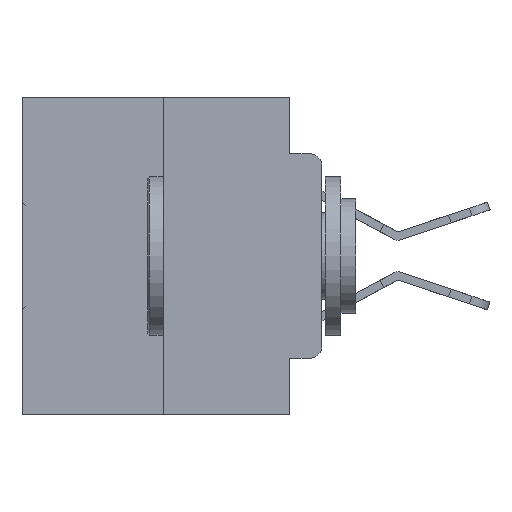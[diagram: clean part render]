
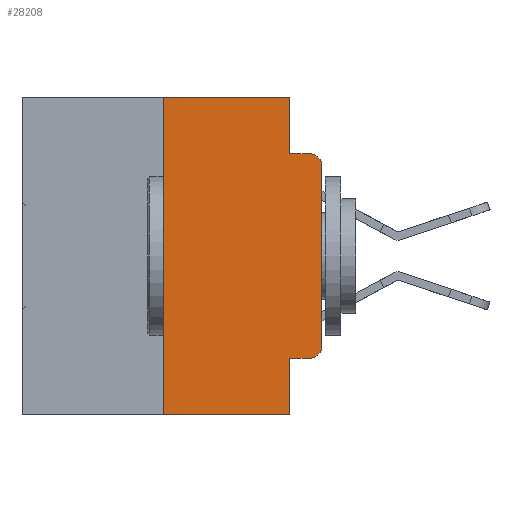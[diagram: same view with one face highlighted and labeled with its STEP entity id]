
A CAD part, left-side view. The second image highlights one B-rep face of the part: STEP entity #28208.
In plain terms, the highlighted planar face has unit normal (-1, 0, 0).
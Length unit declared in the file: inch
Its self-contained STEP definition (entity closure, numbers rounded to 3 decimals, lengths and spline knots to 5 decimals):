
#114 = DIRECTION ( 'NONE',  ( 0., 0., -1. ) ) ;
#362 = EDGE_CURVE ( 'NONE', #10582, #13697, #19929, .T. ) ;
#830 = VERTEX_POINT ( 'NONE', #8700 ) ;
#1329 = LINE ( 'NONE', #29968, #14332 ) ;
#1713 = VERTEX_POINT ( 'NONE', #24439 ) ;
#2024 = CARTESIAN_POINT ( 'NONE',  ( 0., 0., -0.3915 ) ) ;
#2115 = DIRECTION ( 'NONE',  ( 0., 0., -1. ) ) ;
#2784 = EDGE_CURVE ( 'NONE', #21373, #20872, #1329, .T. ) ;
#3033 = DIRECTION ( 'NONE',  ( 1., 0., 0. ) ) ;
#3530 = CARTESIAN_POINT ( 'NONE',  ( 0., 0.051, 0. ) ) ;
#3586 = CARTESIAN_POINT ( 'NONE',  ( 0., 0.051, -0.0885 ) ) ;
#3989 = LINE ( 'NONE', #27292, #23705 ) ;
#3999 = CARTESIAN_POINT ( 'NONE',  ( 0., 0.051, -0.4115 ) ) ;
#5716 = VECTOR ( 'NONE', #10971, 39.37008 ) ;
#5851 = CIRCLE ( 'NONE', #15450, 0.02 ) ;
#6141 = DIRECTION ( 'NONE',  ( 0., -1., 0. ) ) ;
#6340 = VECTOR ( 'NONE', #17680, 39.37008 ) ;
#7231 = CARTESIAN_POINT ( 'NONE',  ( 0., 0.25, -0.5 ) ) ;
#8589 = ORIENTED_EDGE ( 'NONE', *, *, #23967, .T. ) ;
#8700 = CARTESIAN_POINT ( 'NONE',  ( 0., 0.051, -0.4115 ) ) ;
#8953 = ORIENTED_EDGE ( 'NONE', *, *, #32810, .T. ) ;
#9267 = LINE ( 'NONE', #3586, #15259 ) ;
#9735 = VERTEX_POINT ( 'NONE', #19317 ) ;
#9889 = DIRECTION ( 'NONE',  ( -1., 0., 0. ) ) ;
#10582 = VERTEX_POINT ( 'NONE', #7231 ) ;
#10587 = ORIENTED_EDGE ( 'NONE', *, *, #2784, .F. ) ;
#10741 = FACE_OUTER_BOUND ( 'NONE', #18097, .T. ) ;
#10971 = DIRECTION ( 'NONE',  ( 0., 0., -1. ) ) ;
#11123 = DIRECTION ( 'NONE',  ( 0., 0., 1. ) ) ;
#11257 = CARTESIAN_POINT ( 'NONE',  ( 0., 0.051, -0.0885 ) ) ;
#11525 = CARTESIAN_POINT ( 'NONE',  ( 0., 0.25, 0. ) ) ;
#12184 = ORIENTED_EDGE ( 'NONE', *, *, #362, .F. ) ;
#12573 = LINE ( 'NONE', #26244, #5716 ) ;
#12665 = EDGE_CURVE ( 'NONE', #9735, #17681, #5851, .T. ) ;
#13697 = VERTEX_POINT ( 'NONE', #11525 ) ;
#13756 = LINE ( 'NONE', #26394, #15350 ) ;
#14332 = VECTOR ( 'NONE', #114, 39.37008 ) ;
#15259 = VECTOR ( 'NONE', #6141, 39.37008 ) ;
#15350 = VECTOR ( 'NONE', #11123, 39.37008 ) ;
#15360 = EDGE_CURVE ( 'NONE', #10582, #24983, #16429, .T. ) ;
#15450 = AXIS2_PLACEMENT_3D ( 'NONE', #25201, #9889, #27742 ) ;
#15531 = CARTESIAN_POINT ( 'NONE',  ( 0., 0.473, -0.5 ) ) ;
#15731 = VECTOR ( 'NONE', #24563, 39.37008 ) ;
#15901 = PLANE ( 'NONE',  #16919 ) ;
#16429 = LINE ( 'NONE', #15531, #23247 ) ;
#16919 = AXIS2_PLACEMENT_3D ( 'NONE', #26060, #3033, #21022 ) ;
#17575 = DIRECTION ( 'NONE',  ( -1., 0., 0. ) ) ;
#17680 = DIRECTION ( 'NONE',  ( 0., 0., 1. ) ) ;
#17681 = VERTEX_POINT ( 'NONE', #2024 ) ;
#18097 = EDGE_LOOP ( 'NONE', ( #28496, #8953, #30081, #10587, #30868, #12184, #32372, #20541, #8589, #22158 ) ) ;
#19317 = CARTESIAN_POINT ( 'NONE',  ( 0., 0.02, -0.4115 ) ) ;
#19929 = LINE ( 'NONE', #20546, #6340 ) ;
#20541 = ORIENTED_EDGE ( 'NONE', *, *, #30053, .F. ) ;
#20546 = CARTESIAN_POINT ( 'NONE',  ( 0., 0.25, 0. ) ) ;
#20872 = VERTEX_POINT ( 'NONE', #11257 ) ;
#21017 = CARTESIAN_POINT ( 'NONE',  ( 0., 0.051, -0.5 ) ) ;
#21022 = DIRECTION ( 'NONE',  ( 0., 0., -1. ) ) ;
#21373 = VERTEX_POINT ( 'NONE', #3530 ) ;
#22158 = ORIENTED_EDGE ( 'NONE', *, *, #12665, .T. ) ;
#23247 = VECTOR ( 'NONE', #30769, 39.37008 ) ;
#23705 = VECTOR ( 'NONE', #29803, 39.37008 ) ;
#23790 = EDGE_CURVE ( 'NONE', #17681, #27287, #13756, .T. ) ;
#23967 = EDGE_CURVE ( 'NONE', #830, #9735, #29257, .T. ) ;
#24439 = CARTESIAN_POINT ( 'NONE',  ( 0., 0.02, -0.0885 ) ) ;
#24563 = DIRECTION ( 'NONE',  ( 0., -1., 0. ) ) ;
#24607 = EDGE_CURVE ( 'NONE', #13697, #21373, #3989, .T. ) ;
#24983 = VERTEX_POINT ( 'NONE', #21017 ) ;
#25141 = EDGE_CURVE ( 'NONE', #20872, #1713, #9267, .T. ) ;
#25201 = CARTESIAN_POINT ( 'NONE',  ( 0., 0.02, -0.3915 ) ) ;
#26060 = CARTESIAN_POINT ( 'NONE',  ( 0., 0.473, 0. ) ) ;
#26244 = CARTESIAN_POINT ( 'NONE',  ( 0., 0.051, 0. ) ) ;
#26394 = CARTESIAN_POINT ( 'NONE',  ( 0., 0., 0. ) ) ;
#26786 = CIRCLE ( 'NONE', #27916, 0.02 ) ;
#27287 = VERTEX_POINT ( 'NONE', #32526 ) ;
#27292 = CARTESIAN_POINT ( 'NONE',  ( 0., 0.473, 0. ) ) ;
#27742 = DIRECTION ( 'NONE',  ( 0., 0., -1. ) ) ;
#27916 = AXIS2_PLACEMENT_3D ( 'NONE', #32704, #17575, #2115 ) ;
#28208 = ADVANCED_FACE ( 'NONE', ( #10741 ), #15901, .F. ) ;
#28496 = ORIENTED_EDGE ( 'NONE', *, *, #23790, .T. ) ;
#29257 = LINE ( 'NONE', #3999, #15731 ) ;
#29803 = DIRECTION ( 'NONE',  ( 0., -1., 0. ) ) ;
#29968 = CARTESIAN_POINT ( 'NONE',  ( 0., 0.051, 0. ) ) ;
#30053 = EDGE_CURVE ( 'NONE', #830, #24983, #12573, .T. ) ;
#30081 = ORIENTED_EDGE ( 'NONE', *, *, #25141, .F. ) ;
#30769 = DIRECTION ( 'NONE',  ( 0., -1., 0. ) ) ;
#30868 = ORIENTED_EDGE ( 'NONE', *, *, #24607, .F. ) ;
#32372 = ORIENTED_EDGE ( 'NONE', *, *, #15360, .T. ) ;
#32526 = CARTESIAN_POINT ( 'NONE',  ( 0., 0., -0.1085 ) ) ;
#32704 = CARTESIAN_POINT ( 'NONE',  ( 0., 0.02, -0.1085 ) ) ;
#32810 = EDGE_CURVE ( 'NONE', #27287, #1713, #26786, .T. ) ;
